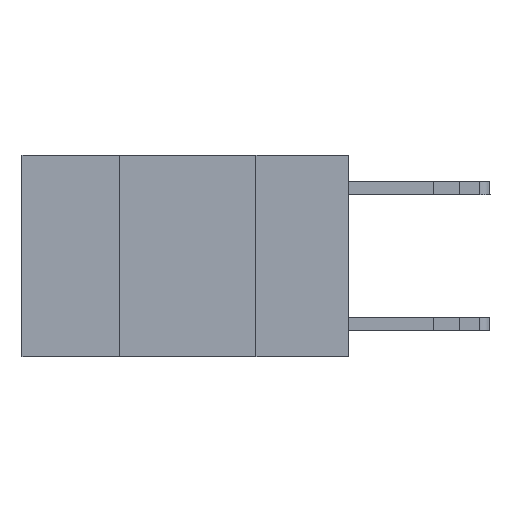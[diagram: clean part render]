
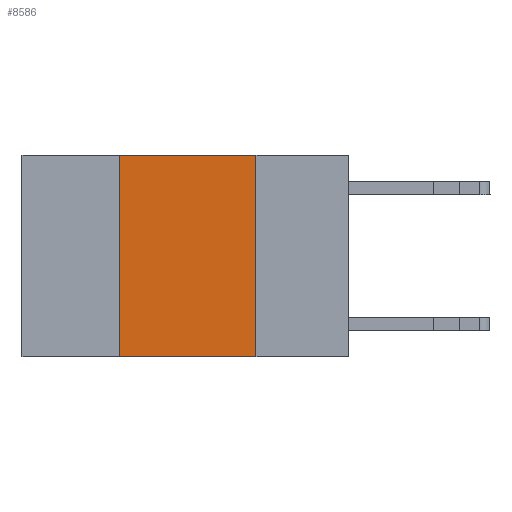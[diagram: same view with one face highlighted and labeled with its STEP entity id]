
A CAD part, left-side view. The second image highlights one B-rep face of the part: STEP entity #8586.
In plain terms, the highlighted planar face has unit normal (-1, 0, 0).
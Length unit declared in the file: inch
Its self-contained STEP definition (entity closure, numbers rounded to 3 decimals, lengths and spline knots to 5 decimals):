
#91 = EDGE_CURVE ( 'NONE', #12235, #11354, #5874, .T. ) ;
#1154 = ORIENTED_EDGE ( 'NONE', *, *, #91, .F. ) ;
#1612 = LINE ( 'NONE', #10234, #6553 ) ;
#2591 = EDGE_CURVE ( 'NONE', #12235, #13580, #1612, .T. ) ;
#2871 = EDGE_CURVE ( 'NONE', #11354, #6268, #13072, .T. ) ;
#2969 = AXIS2_PLACEMENT_3D ( 'NONE', #2996, #11386, #7319 ) ;
#2996 = CARTESIAN_POINT ( 'NONE',  ( 0., 0.6, 0. ) ) ;
#3134 = CARTESIAN_POINT ( 'NONE',  ( 0., 0.17, -0.37 ) ) ;
#3301 = EDGE_LOOP ( 'NONE', ( #7704, #13370, #1154, #6078 ) ) ;
#3599 = CARTESIAN_POINT ( 'NONE',  ( 0., 0.42, 0. ) ) ;
#4075 = VECTOR ( 'NONE', #12205, 39.37008 ) ;
#4736 = CARTESIAN_POINT ( 'NONE',  ( 0., 0.17, 0. ) ) ;
#5279 = EDGE_CURVE ( 'NONE', #6268, #13580, #5359, .T. ) ;
#5359 = LINE ( 'NONE', #12763, #5405 ) ;
#5405 = VECTOR ( 'NONE', #13992, 39.37008 ) ;
#5874 = LINE ( 'NONE', #3599, #4075 ) ;
#6078 = ORIENTED_EDGE ( 'NONE', *, *, #2591, .T. ) ;
#6268 = VERTEX_POINT ( 'NONE', #4736 ) ;
#6437 = CARTESIAN_POINT ( 'NONE',  ( 0., 0.6, 0. ) ) ;
#6553 = VECTOR ( 'NONE', #12431, 39.37008 ) ;
#7200 = VECTOR ( 'NONE', #10718, 39.37008 ) ;
#7319 = DIRECTION ( 'NONE',  ( 0., 0., -1. ) ) ;
#7704 = ORIENTED_EDGE ( 'NONE', *, *, #5279, .F. ) ;
#8228 = FACE_OUTER_BOUND ( 'NONE', #3301, .T. ) ;
#8372 = PLANE ( 'NONE',  #2969 ) ;
#8586 = ADVANCED_FACE ( 'NONE', ( #8228 ), #8372, .F. ) ;
#10234 = CARTESIAN_POINT ( 'NONE',  ( 0., 0.6, -0.37 ) ) ;
#10718 = DIRECTION ( 'NONE',  ( 0., -1., 0. ) ) ;
#11313 = CARTESIAN_POINT ( 'NONE',  ( 0., 0.42, -0.37 ) ) ;
#11354 = VERTEX_POINT ( 'NONE', #12489 ) ;
#11386 = DIRECTION ( 'NONE',  ( 1., 0., 0. ) ) ;
#12205 = DIRECTION ( 'NONE',  ( 0., 0., 1. ) ) ;
#12235 = VERTEX_POINT ( 'NONE', #11313 ) ;
#12431 = DIRECTION ( 'NONE',  ( 0., -1., 0. ) ) ;
#12489 = CARTESIAN_POINT ( 'NONE',  ( 0., 0.42, 0. ) ) ;
#12763 = CARTESIAN_POINT ( 'NONE',  ( 0., 0.17, 0. ) ) ;
#13072 = LINE ( 'NONE', #6437, #7200 ) ;
#13370 = ORIENTED_EDGE ( 'NONE', *, *, #2871, .F. ) ;
#13580 = VERTEX_POINT ( 'NONE', #3134 ) ;
#13992 = DIRECTION ( 'NONE',  ( 0., 0., -1. ) ) ;
